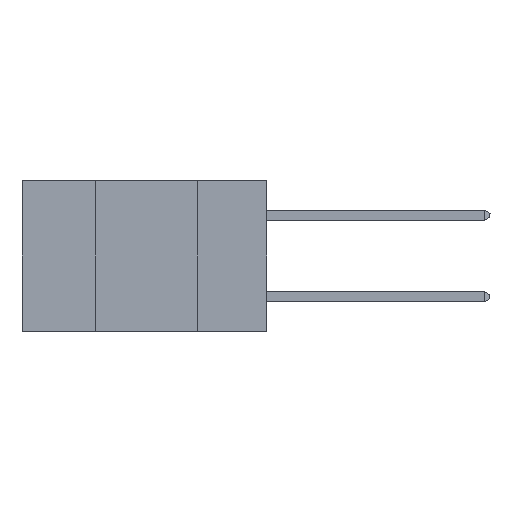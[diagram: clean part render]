
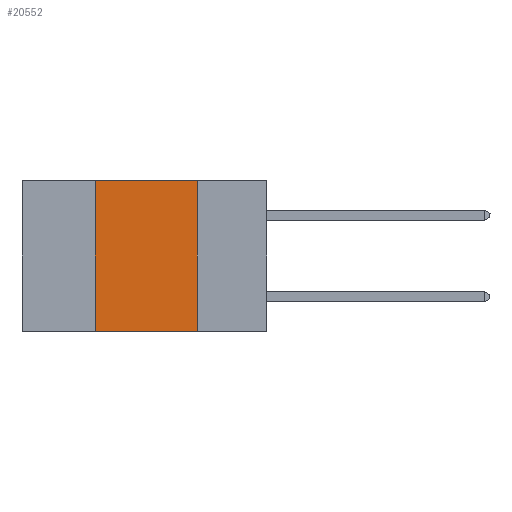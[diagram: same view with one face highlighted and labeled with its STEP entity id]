
A CAD part, left-side view. The second image highlights one B-rep face of the part: STEP entity #20552.
In plain terms, the highlighted planar face has unit normal (-1, 0, 0).
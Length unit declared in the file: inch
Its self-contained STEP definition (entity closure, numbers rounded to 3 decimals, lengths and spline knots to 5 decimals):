
#167 = VECTOR ( 'NONE', #19190, 39.37008 ) ;
#764 = LINE ( 'NONE', #10566, #1743 ) ;
#914 = DIRECTION ( 'NONE',  ( 0., -1., 0. ) ) ;
#1638 = FACE_OUTER_BOUND ( 'NONE', #9806, .T. ) ;
#1743 = VECTOR ( 'NONE', #914, 39.37008 ) ;
#2834 = VERTEX_POINT ( 'NONE', #6777 ) ;
#3172 = CARTESIAN_POINT ( 'NONE',  ( 0., 0.42, -0.37 ) ) ;
#3582 = CARTESIAN_POINT ( 'NONE',  ( 0., 0.6, 0. ) ) ;
#3994 = DIRECTION ( 'NONE',  ( 0., 0., -1. ) ) ;
#6777 = CARTESIAN_POINT ( 'NONE',  ( 0., 0.17, 0. ) ) ;
#6871 = LINE ( 'NONE', #21569, #167 ) ;
#7694 = EDGE_CURVE ( 'NONE', #2834, #12367, #30867, .T. ) ;
#7749 = VECTOR ( 'NONE', #3994, 39.37008 ) ;
#9129 = CARTESIAN_POINT ( 'NONE',  ( 0., 0.42, 0. ) ) ;
#9806 = EDGE_LOOP ( 'NONE', ( #17429, #27010, #16174, #10571 ) ) ;
#10137 = VERTEX_POINT ( 'NONE', #3172 ) ;
#10566 = CARTESIAN_POINT ( 'NONE',  ( 0., 0.6, -0.37 ) ) ;
#10571 = ORIENTED_EDGE ( 'NONE', *, *, #23249, .T. ) ;
#11649 = EDGE_CURVE ( 'NONE', #11693, #2834, #6871, .T. ) ;
#11693 = VERTEX_POINT ( 'NONE', #9129 ) ;
#12367 = VERTEX_POINT ( 'NONE', #27412 ) ;
#16062 = AXIS2_PLACEMENT_3D ( 'NONE', #3582, #23711, #30449 ) ;
#16174 = ORIENTED_EDGE ( 'NONE', *, *, #30083, .F. ) ;
#17429 = ORIENTED_EDGE ( 'NONE', *, *, #7694, .F. ) ;
#19190 = DIRECTION ( 'NONE',  ( 0., -1., 0. ) ) ;
#20552 = ADVANCED_FACE ( 'NONE', ( #1638 ), #20858, .F. ) ;
#20858 = PLANE ( 'NONE',  #16062 ) ;
#21569 = CARTESIAN_POINT ( 'NONE',  ( 0., 0.6, 0. ) ) ;
#23249 = EDGE_CURVE ( 'NONE', #10137, #12367, #764, .T. ) ;
#23336 = LINE ( 'NONE', #25889, #26489 ) ;
#23711 = DIRECTION ( 'NONE',  ( 1., 0., 0. ) ) ;
#25889 = CARTESIAN_POINT ( 'NONE',  ( 0., 0.42, 0. ) ) ;
#25900 = CARTESIAN_POINT ( 'NONE',  ( 0., 0.17, 0. ) ) ;
#26489 = VECTOR ( 'NONE', #30539, 39.37008 ) ;
#27010 = ORIENTED_EDGE ( 'NONE', *, *, #11649, .F. ) ;
#27412 = CARTESIAN_POINT ( 'NONE',  ( 0., 0.17, -0.37 ) ) ;
#30083 = EDGE_CURVE ( 'NONE', #10137, #11693, #23336, .T. ) ;
#30449 = DIRECTION ( 'NONE',  ( 0., 0., -1. ) ) ;
#30539 = DIRECTION ( 'NONE',  ( 0., 0., 1. ) ) ;
#30867 = LINE ( 'NONE', #25900, #7749 ) ;
